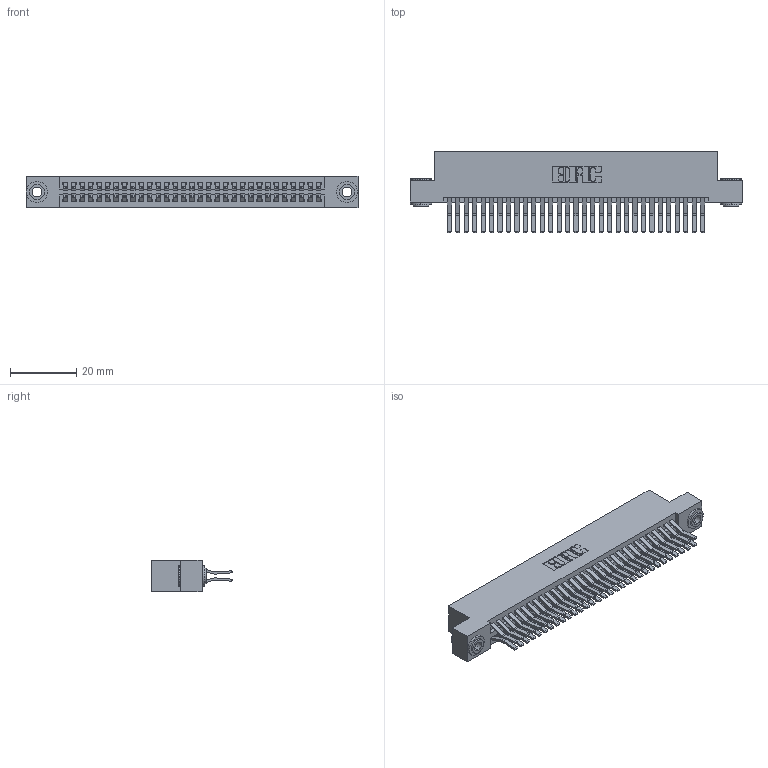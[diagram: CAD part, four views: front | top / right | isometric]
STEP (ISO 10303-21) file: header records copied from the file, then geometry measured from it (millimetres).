
FILE_DESCRIPTION (( 'STEP AP203' ), '1' );
FILE_NAME ('395-062-560-203.STEP', '2019-10-23T17:16:22', ( '' ), ( '' ), 'SwSTEP 2.0', 'SolidWorks 2016', '' );
FILE_SCHEMA (( 'CONFIG_CONTROL_DESIGN' ));
Length unit declared in the file: inch
Products named in the file (4): 345-292-001_560 Tail; 345-250-002_345-250-002-102; 395-062-560-203; 345 Part_Flush Mounting Lugs - 0.156 Dia-TH
Assembly tree (65 placements, depth 2):
  395-062-560-203
    345 Part_Flush Mounting Lugs - 0.156 Dia-TH
    345-292-001_560 Tail  x62
    345-250-002_345-250-002-102  x2
Bounding box: 99.95 x 24.45 x 9.4 mm (x, y, z)
Volume: 10032.8 mm3; surface area: 15867.2 mm2
Topology: 65 solids, 65 shells, 3388 faces, 10027 edges, 6598 vertices
Faces by surface type: plane 2136, cylinder 1244, cone 8
Entity records: 26542 total; most frequent: CARTESIAN_POINT 4435, ORIENTED_EDGE 4362, DIRECTION 3959, EDGE_CURVE 2181, LINE 1897, VECTOR 1897, VERTEX_POINT 1450, AXIS2_PLACEMENT_3D 1031
